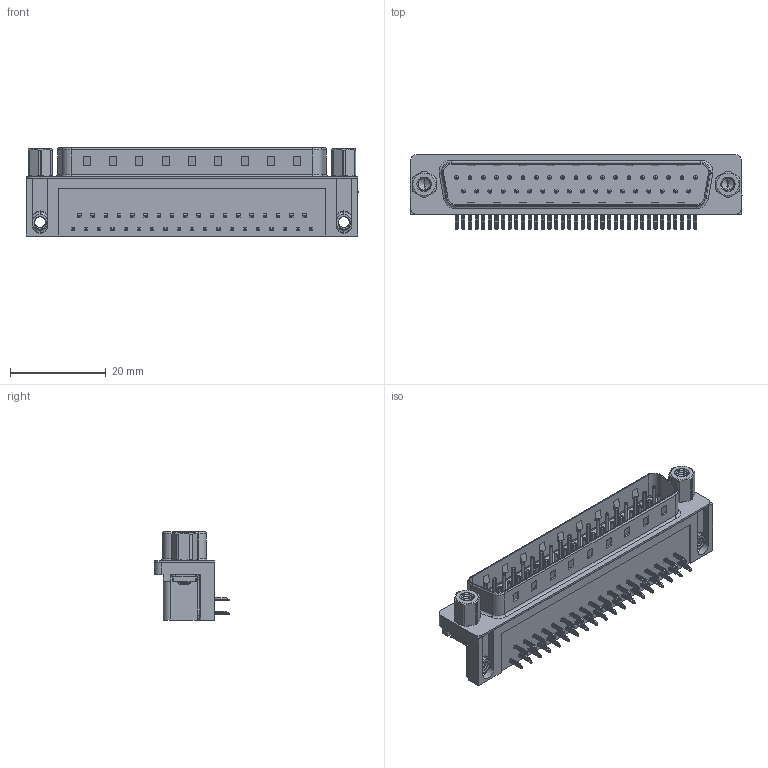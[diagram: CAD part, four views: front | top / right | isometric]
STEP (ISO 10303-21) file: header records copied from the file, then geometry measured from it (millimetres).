
FILE_DESCRIPTION (( 'STEP AP203' ), '1' );
FILE_NAME ('621-037-660-556.STEP', '2019-11-19T11:06:26', ( '' ), ( '' ), 'SwSTEP 2.0', 'SolidWorks 2016', '' );
FILE_SCHEMA (( 'CONFIG_CONTROL_DESIGN' ));
Length unit declared in the file: millimetre
Products named in the file (8): 621 4-40 Threaded Board Mount; 621 Housing_37 Socket; 621 Contact Bottom; 621 M3 Hex Standoff 5; 621 M3 Threaded Rivet; 621-037-660-556; 621 Contact Top; 621 Shell_37 Socket
Assembly tree (45 placements, depth 2):
  621-037-660-556
    621 Housing_37 Socket
    621 Shell_37 Socket
    621 Contact Bottom  x18
    621 Contact Top  x19
    621 4-40 Threaded Board Mount  x2
    621 M3 Threaded Rivet  x2
    621 M3 Hex Standoff 5  x2
Bounding box: 69.4 x 15.73 x 18.4 mm (x, y, z)
Volume: 8872 mm3; surface area: 10705.7 mm2
Topology: 45 solids, 45 shells, 3377 faces, 8395 edges, 5191 vertices
Faces by surface type: plane 2035, cylinder 1023, torus 265, cone 30, bspline 24
Entity records: 33651 total; most frequent: CARTESIAN_POINT 10635, ORIENTED_EDGE 4382, DIRECTION 4373, EDGE_CURVE 2191, VECTOR 1483, LINE 1483, AXIS2_PLACEMENT_3D 1445, VERTEX_POINT 1414
